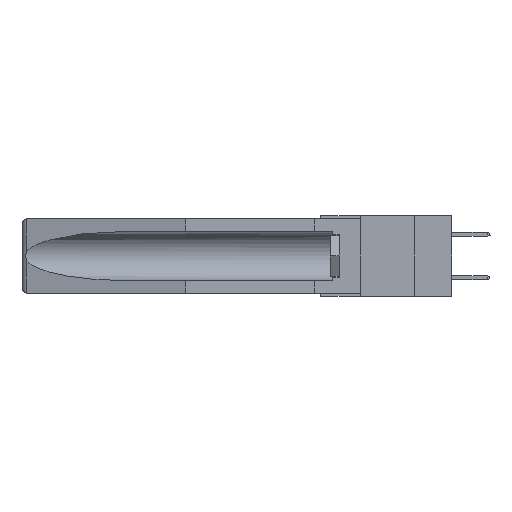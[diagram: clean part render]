
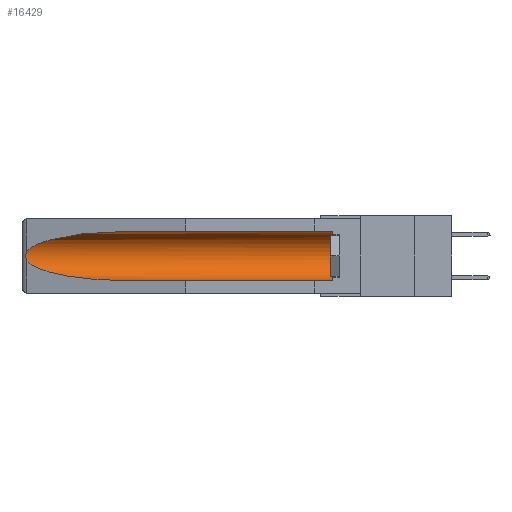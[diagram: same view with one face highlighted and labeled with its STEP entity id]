
A CAD part, left-side view. The second image highlights one B-rep face of the part: STEP entity #16429.
In plain terms, the highlighted cylindrical face has radius 2.857 mm (diameter 5.715 mm), a partial arc.
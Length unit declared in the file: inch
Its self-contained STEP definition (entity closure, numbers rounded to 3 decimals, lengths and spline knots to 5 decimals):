
#918 = DIRECTION ( 'NONE',  ( 0., 0., 1. ) ) ;
#979 = DIRECTION ( 'NONE',  ( 0., 1., 0. ) ) ;
#1868 = CARTESIAN_POINT ( 'NONE',  ( 0.155, 1.07973, -0.284 ) ) ;
#2062 = CARTESIAN_POINT ( 'NONE',  ( 0.25451, 1.48313, -0.24835 ) ) ;
#2188 = EDGE_CURVE ( 'NONE', #7710, #3369, #16819, .T. ) ;
#2373 = DIRECTION ( 'NONE',  ( 0., -1., 0. ) ) ;
#2570 = ORIENTED_EDGE ( 'NONE', *, *, #8531, .T. ) ;
#2732 = B_SPLINE_CURVE_WITH_KNOTS ( 'NONE', 3,
 ( #4681, #14494, #15921, #7393, #6101, #17369, #16158, #7516, #8940, #3303 ),
 .UNSPECIFIED., .F., .F.,
 ( 4, 2, 2, 2, 4 ),
 ( 0., 0.00029, 0.00058, 0.00087, 0.00117 ),
 .UNSPECIFIED. ) ;
#3279 = AXIS2_PLACEMENT_3D ( 'NONE', #3729, #979, #918 ) ;
#3303 = CARTESIAN_POINT ( 'NONE',  ( 0.26537, 1.52718, -0.19328 ) ) ;
#3369 = VERTEX_POINT ( 'NONE', #8102 ) ;
#3448 = LINE ( 'NONE', #9922, #16365 ) ;
#3729 = CARTESIAN_POINT ( 'NONE',  ( 0.155, -0.30754, -0.1715 ) ) ;
#3785 = DIRECTION ( 'NONE',  ( 0., 1., 0. ) ) ;
#3904 = ORIENTED_EDGE ( 'NONE', *, *, #13297, .T. ) ;
#4669 = ORIENTED_EDGE ( 'NONE', *, *, #15845, .T. ) ;
#4681 = CARTESIAN_POINT ( 'NONE',  ( 0.26537, 1.52718, -0.14972 ) ) ;
#4728 = CARTESIAN_POINT ( 'NONE',  ( 0.26537, 1.52718, -0.19328 ) ) ;
#4764 = CARTESIAN_POINT ( 'NONE',  ( 0.155, 1.07973, -0.059 ) ) ;
#5206 = ORIENTED_EDGE ( 'NONE', *, *, #14648, .T. ) ;
#5220 = DIRECTION ( 'NONE',  ( 0., 0., 1. ) ) ;
#5428 = CYLINDRICAL_SURFACE ( 'NONE', #3279, 0.1125 ) ;
#5563 = VERTEX_POINT ( 'NONE', #18113 ) ;
#6032 = CIRCLE ( 'NONE', #17937, 0.1125 ) ;
#6101 = CARTESIAN_POINT ( 'NONE',  ( 0.2675, 1.53308, -0.16763 ) ) ;
#6232 = VERTEX_POINT ( 'NONE', #4764 ) ;
#6279 = CARTESIAN_POINT ( 'NONE',  ( 0.21114, 1.30732, -0.284 ) ) ;
#6418 = VERTEX_POINT ( 'NONE', #11542 ) ;
#6580 = VERTEX_POINT ( 'NONE', #8937 ) ;
#7201 = FACE_OUTER_BOUND ( 'NONE', #15838, .T. ) ;
#7393 = CARTESIAN_POINT ( 'NONE',  ( 0.2673, 1.5327, -0.16383 ) ) ;
#7516 = CARTESIAN_POINT ( 'NONE',  ( 0.26655, 1.53094, -0.18657 ) ) ;
#7710 = VERTEX_POINT ( 'NONE', #18324 ) ;
#8102 = CARTESIAN_POINT ( 'NONE',  ( 0.155, 1.07973, -0.284 ) ) ;
#8464 = ORIENTED_EDGE ( 'NONE', *, *, #2188, .F. ) ;
#8531 = EDGE_CURVE ( 'NONE', #6580, #5563, #2732, .T. ) ;
#8937 = CARTESIAN_POINT ( 'NONE',  ( 0.26537, 1.52718, -0.14972 ) ) ;
#8940 = CARTESIAN_POINT ( 'NONE',  ( 0.26597, 1.5296, -0.19026 ) ) ;
#9056 = CARTESIAN_POINT ( 'NONE',  ( 0.21114, 1.30732, -0.059 ) ) ;
#9231 = VECTOR ( 'NONE', #3785, 39.37008 ) ;
#9922 = CARTESIAN_POINT ( 'NONE',  ( 0.155, -0.30754, -0.059 ) ) ;
#10921 = EDGE_CURVE ( 'NONE', #6232, #6580, #18143, .T. ) ;
#11542 = CARTESIAN_POINT ( 'NONE',  ( 0.155, 0.126, -0.059 ) ) ;
#12004 = CARTESIAN_POINT ( 'NONE',  ( 0.25451, 1.48313, -0.09465 ) ) ;
#13297 = EDGE_CURVE ( 'NONE', #7710, #6418, #6032, .T. ) ;
#13736 = CARTESIAN_POINT ( 'NONE',  ( 0.155, -0.30754, -0.284 ) ) ;
#14494 = CARTESIAN_POINT ( 'NONE',  ( 0.26597, 1.52961, -0.15275 ) ) ;
#14648 = EDGE_CURVE ( 'NONE', #5563, #3369, #15937, .T. ) ;
#14801 = CARTESIAN_POINT ( 'NONE',  ( 0.155, 1.07973, -0.059 ) ) ;
#15113 = CARTESIAN_POINT ( 'NONE',  ( 0.155, 0.126, -0.1715 ) ) ;
#15832 = DIRECTION ( 'NONE',  ( 0., 1., 0. ) ) ;
#15838 = EDGE_LOOP ( 'NONE', ( #16265, #2570, #5206, #8464, #3904, #4669 ) ) ;
#15845 = EDGE_CURVE ( 'NONE', #6418, #6232, #3448, .T. ) ;
#15921 = CARTESIAN_POINT ( 'NONE',  ( 0.26654, 1.53092, -0.15636 ) ) ;
#15937 =( BOUNDED_CURVE ( )  B_SPLINE_CURVE ( 3, ( #4728, #2062, #6279, #1868 ),
 .UNSPECIFIED., .F., .F. ) 
 B_SPLINE_CURVE_WITH_KNOTS ( ( 4, 4 ),
 ( 0.1948, 1.5708 ),
 .UNSPECIFIED. ) 
 CURVE ( )  GEOMETRIC_REPRESENTATION_ITEM ( )  RATIONAL_B_SPLINE_CURVE ( ( 1., 0.848, 0.848, 1. ) ) 
 REPRESENTATION_ITEM ( '' )  );
#16158 = CARTESIAN_POINT ( 'NONE',  ( 0.2673, 1.53269, -0.17917 ) ) ;
#16265 = ORIENTED_EDGE ( 'NONE', *, *, #10921, .T. ) ;
#16365 = VECTOR ( 'NONE', #15832, 39.37008 ) ;
#16429 = ADVANCED_FACE ( 'NONE', ( #7201 ), #5428, .F. ) ;
#16819 = LINE ( 'NONE', #13736, #9231 ) ;
#17369 = CARTESIAN_POINT ( 'NONE',  ( 0.2675, 1.53308, -0.17534 ) ) ;
#17731 = CARTESIAN_POINT ( 'NONE',  ( 0.26537, 1.52718, -0.14972 ) ) ;
#17937 = AXIS2_PLACEMENT_3D ( 'NONE', #15113, #2373, #5220 ) ;
#18113 = CARTESIAN_POINT ( 'NONE',  ( 0.26537, 1.52718, -0.19328 ) ) ;
#18143 =( BOUNDED_CURVE ( )  B_SPLINE_CURVE ( 3, ( #14801, #9056, #12004, #17731 ),
 .UNSPECIFIED., .F., .F. ) 
 B_SPLINE_CURVE_WITH_KNOTS ( ( 4, 4 ),
 ( 4.71239, 6.08839 ),
 .UNSPECIFIED. ) 
 CURVE ( )  GEOMETRIC_REPRESENTATION_ITEM ( )  RATIONAL_B_SPLINE_CURVE ( ( 1., 0.848, 0.848, 1. ) ) 
 REPRESENTATION_ITEM ( '' )  );
#18324 = CARTESIAN_POINT ( 'NONE',  ( 0.155, 0.126, -0.284 ) ) ;
